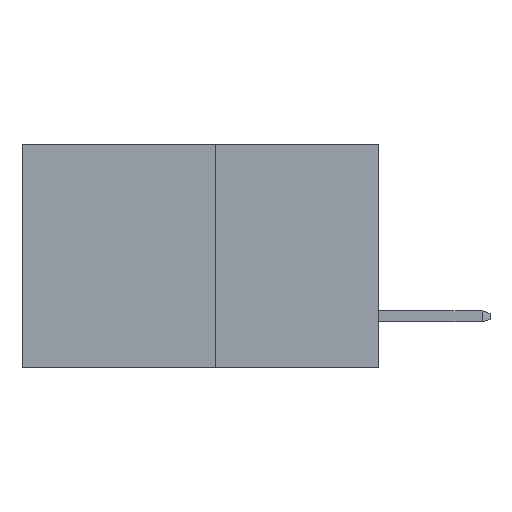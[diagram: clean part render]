
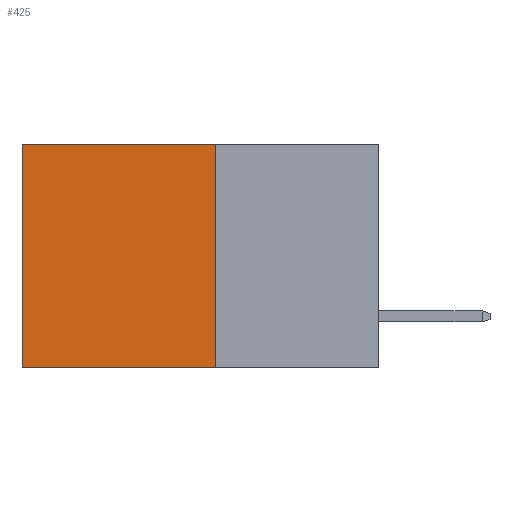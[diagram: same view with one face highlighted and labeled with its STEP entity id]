
A CAD part, left-side view. The second image highlights one B-rep face of the part: STEP entity #425.
In plain terms, the highlighted planar face has unit normal (-1, 0, 0).
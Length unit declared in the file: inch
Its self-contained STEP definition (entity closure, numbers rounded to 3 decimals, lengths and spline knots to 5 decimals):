
#261 = ORIENTED_EDGE ( 'NONE', *, *, #6016, .F. ) ;
#425 = ADVANCED_FACE ( 'NONE', ( #1823 ), #3711, .F. ) ;
#1140 = VERTEX_POINT ( 'NONE', #2169 ) ;
#1335 = EDGE_CURVE ( 'NONE', #1140, #3251, #5679, .T. ) ;
#1675 = DIRECTION ( 'NONE',  ( 0., 0., -1. ) ) ;
#1823 = FACE_OUTER_BOUND ( 'NONE', #3861, .T. ) ;
#2108 = AXIS2_PLACEMENT_3D ( 'NONE', #4555, #5906, #3419 ) ;
#2115 = DIRECTION ( 'NONE',  ( 0., 1., 0. ) ) ;
#2169 = CARTESIAN_POINT ( 'NONE',  ( 0.277, 0.27, 0. ) ) ;
#2222 = LINE ( 'NONE', #3985, #4060 ) ;
#2234 = ORIENTED_EDGE ( 'NONE', *, *, #1335, .T. ) ;
#2359 = CARTESIAN_POINT ( 'NONE',  ( 0.277, 0.27, -0.37 ) ) ;
#3251 = VERTEX_POINT ( 'NONE', #6342 ) ;
#3254 = EDGE_CURVE ( 'NONE', #4818, #5546, #5903, .T. ) ;
#3419 = DIRECTION ( 'NONE',  ( 0., 0., -1. ) ) ;
#3632 = CARTESIAN_POINT ( 'NONE',  ( 0.277, 0.27, -0.37 ) ) ;
#3711 = PLANE ( 'NONE',  #2108 ) ;
#3850 = ORIENTED_EDGE ( 'NONE', *, *, #7316, .T. ) ;
#3861 = EDGE_LOOP ( 'NONE', ( #3850, #5545, #261, #2234 ) ) ;
#3954 = DIRECTION ( 'NONE',  ( 0., 0., -1. ) ) ;
#3971 = LINE ( 'NONE', #2359, #5652 ) ;
#3985 = CARTESIAN_POINT ( 'NONE',  ( 0.277, 0.59, -0.37 ) ) ;
#4060 = VECTOR ( 'NONE', #3954, 39.37008 ) ;
#4229 = VECTOR ( 'NONE', #6582, 39.37008 ) ;
#4555 = CARTESIAN_POINT ( 'NONE',  ( 0.277, 0.27, -0.37 ) ) ;
#4818 = VERTEX_POINT ( 'NONE', #3632 ) ;
#5545 = ORIENTED_EDGE ( 'NONE', *, *, #3254, .F. ) ;
#5546 = VERTEX_POINT ( 'NONE', #7428 ) ;
#5652 = VECTOR ( 'NONE', #1675, 39.37008 ) ;
#5679 = LINE ( 'NONE', #6606, #4229 ) ;
#5903 = LINE ( 'NONE', #6108, #6259 ) ;
#5906 = DIRECTION ( 'NONE',  ( 1., 0., 0. ) ) ;
#6016 = EDGE_CURVE ( 'NONE', #1140, #4818, #3971, .T. ) ;
#6108 = CARTESIAN_POINT ( 'NONE',  ( 0.277, 0.27, -0.37 ) ) ;
#6259 = VECTOR ( 'NONE', #2115, 39.37008 ) ;
#6342 = CARTESIAN_POINT ( 'NONE',  ( 0.277, 0.59, 0. ) ) ;
#6582 = DIRECTION ( 'NONE',  ( 0., 1., 0. ) ) ;
#6606 = CARTESIAN_POINT ( 'NONE',  ( 0.277, 0.27, 0. ) ) ;
#7316 = EDGE_CURVE ( 'NONE', #3251, #5546, #2222, .T. ) ;
#7428 = CARTESIAN_POINT ( 'NONE',  ( 0.277, 0.59, -0.37 ) ) ;
